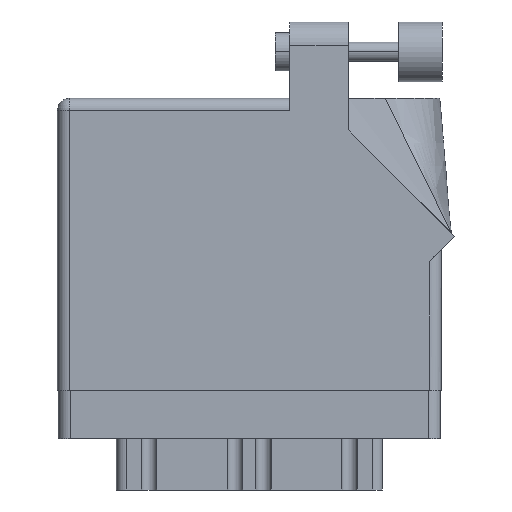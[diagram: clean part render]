
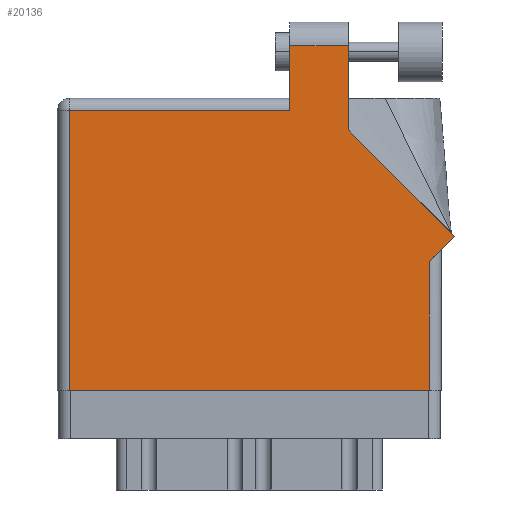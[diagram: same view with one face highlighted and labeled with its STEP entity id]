
A CAD part, front view. The second image highlights one B-rep face of the part: STEP entity #20136.
In plain terms, the highlighted face is planar.
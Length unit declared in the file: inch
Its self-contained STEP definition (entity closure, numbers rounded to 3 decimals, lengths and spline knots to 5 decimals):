
#296 = VERTEX_POINT ( 'NONE', #29452 ) ;
#819 = ORIENTED_EDGE ( 'NONE', *, *, #18401, .T. ) ;
#1143 = PLANE ( 'NONE',  #2238 ) ;
#1325 = VECTOR ( 'NONE', #16028, 39.37008 ) ;
#1350 = DIRECTION ( 'NONE',  ( -1., 0., 0. ) ) ;
#2117 = VECTOR ( 'NONE', #21336, 39.37008 ) ;
#2238 = AXIS2_PLACEMENT_3D ( 'NONE', #15175, #3336, #22206 ) ;
#2289 = CARTESIAN_POINT ( 'NONE',  ( 2.01, 0.737, 0. ) ) ;
#2433 = DIRECTION ( 'NONE',  ( 0., -1., 0. ) ) ;
#3134 = LINE ( 'NONE', #3281, #13833 ) ;
#3281 = CARTESIAN_POINT ( 'NONE',  ( 0., 0., 0. ) ) ;
#3336 = DIRECTION ( 'NONE',  ( 0., 0., -1. ) ) ;
#4710 = CARTESIAN_POINT ( 'NONE',  ( 1.948, 0., 0. ) ) ;
#5114 = ORIENTED_EDGE ( 'NONE', *, *, #14555, .T. ) ;
#5416 = CARTESIAN_POINT ( 'NONE',  ( 1.524, 1.36442, 0. ) ) ;
#7023 = EDGE_CURVE ( 'NONE', #10061, #24584, #21172, .T. ) ;
#7038 = CARTESIAN_POINT ( 'NONE',  ( 1.217, 1.468, 0. ) ) ;
#7581 = ORIENTED_EDGE ( 'NONE', *, *, #28350, .T. ) ;
#8056 = CARTESIAN_POINT ( 'NONE',  ( 1.217, 1.805, 0. ) ) ;
#9410 = LINE ( 'NONE', #28465, #15204 ) ;
#9479 = VERTEX_POINT ( 'NONE', #16394 ) ;
#9563 = DIRECTION ( 'NONE',  ( -1., 0., 0. ) ) ;
#10061 = VERTEX_POINT ( 'NONE', #12580 ) ;
#10605 = DIRECTION ( 'NONE',  ( -0.707, 0.707, 0. ) ) ;
#10945 = EDGE_CURVE ( 'NONE', #30855, #10061, #15712, .T. ) ;
#12081 = LINE ( 'NONE', #16476, #12684 ) ;
#12106 = LINE ( 'NONE', #5416, #21195 ) ;
#12580 = CARTESIAN_POINT ( 'NONE',  ( 1.948, 0.675, 0. ) ) ;
#12672 = FACE_OUTER_BOUND ( 'NONE', #29755, .T. ) ;
#12684 = VECTOR ( 'NONE', #2433, 39.37008 ) ;
#13103 = CARTESIAN_POINT ( 'NONE',  ( 2.08071, 0.80771, 0. ) ) ;
#13833 = VECTOR ( 'NONE', #22327, 39.37008 ) ;
#13899 = ORIENTED_EDGE ( 'NONE', *, *, #26778, .T. ) ;
#14131 = DIRECTION ( 'NONE',  ( 0., -1., 0. ) ) ;
#14555 = EDGE_CURVE ( 'NONE', #25944, #30855, #3134, .T. ) ;
#15175 = CARTESIAN_POINT ( 'NONE',  ( 0., 1.53, 0. ) ) ;
#15204 = VECTOR ( 'NONE', #9563, 39.37008 ) ;
#15604 = LINE ( 'NONE', #13103, #29050 ) ;
#15712 = LINE ( 'NONE', #18375, #1325 ) ;
#16028 = DIRECTION ( 'NONE',  ( 0., 1., 0. ) ) ;
#16394 = CARTESIAN_POINT ( 'NONE',  ( 1.217, 1.805, 0. ) ) ;
#16476 = CARTESIAN_POINT ( 'NONE',  ( 0.062, 0., 0. ) ) ;
#16487 = LINE ( 'NONE', #26012, #23234 ) ;
#17154 = CARTESIAN_POINT ( 'NONE',  ( 1.524, 1.36442, 0. ) ) ;
#17431 = CARTESIAN_POINT ( 'NONE',  ( 1.524, 1.805, 0. ) ) ;
#17796 = EDGE_CURVE ( 'NONE', #24463, #17862, #12106, .T. ) ;
#17862 = VERTEX_POINT ( 'NONE', #17431 ) ;
#17958 = CARTESIAN_POINT ( 'NONE',  ( 2.08071, 0.80771, 0. ) ) ;
#18375 = CARTESIAN_POINT ( 'NONE',  ( 1.948, 0.737, 0. ) ) ;
#18401 = EDGE_CURVE ( 'NONE', #9479, #18559, #16487, .T. ) ;
#18559 = VERTEX_POINT ( 'NONE', #7038 ) ;
#20136 = ADVANCED_FACE ( 'NONE', ( #12672 ), #1143, .F. ) ;
#20399 = LINE ( 'NONE', #8056, #30310 ) ;
#20962 = EDGE_CURVE ( 'NONE', #17862, #9479, #20399, .T. ) ;
#21172 = LINE ( 'NONE', #2289, #2117 ) ;
#21195 = VECTOR ( 'NONE', #21956, 39.37008 ) ;
#21336 = DIRECTION ( 'NONE',  ( 0.707, 0.707, 0. ) ) ;
#21956 = DIRECTION ( 'NONE',  ( 0., 1., 0. ) ) ;
#22110 = CARTESIAN_POINT ( 'NONE',  ( 0.062, 0., 0. ) ) ;
#22206 = DIRECTION ( 'NONE',  ( -1., 0., 0. ) ) ;
#22327 = DIRECTION ( 'NONE',  ( 1., 0., 0. ) ) ;
#23234 = VECTOR ( 'NONE', #14131, 39.37008 ) ;
#23463 = ORIENTED_EDGE ( 'NONE', *, *, #7023, .T. ) ;
#24463 = VERTEX_POINT ( 'NONE', #17154 ) ;
#24584 = VERTEX_POINT ( 'NONE', #17958 ) ;
#24639 = EDGE_CURVE ( 'NONE', #24584, #24463, #15604, .T. ) ;
#25713 = ORIENTED_EDGE ( 'NONE', *, *, #20962, .T. ) ;
#25856 = ORIENTED_EDGE ( 'NONE', *, *, #10945, .T. ) ;
#25882 = ORIENTED_EDGE ( 'NONE', *, *, #17796, .T. ) ;
#25944 = VERTEX_POINT ( 'NONE', #22110 ) ;
#26012 = CARTESIAN_POINT ( 'NONE',  ( 1.217, 1.53, 0. ) ) ;
#26778 = EDGE_CURVE ( 'NONE', #296, #25944, #12081, .T. ) ;
#28350 = EDGE_CURVE ( 'NONE', #18559, #296, #9410, .T. ) ;
#28465 = CARTESIAN_POINT ( 'NONE',  ( 0., 1.468, 0. ) ) ;
#29050 = VECTOR ( 'NONE', #10605, 39.37008 ) ;
#29452 = CARTESIAN_POINT ( 'NONE',  ( 0.062, 1.468, 0. ) ) ;
#29755 = EDGE_LOOP ( 'NONE', ( #25882, #25713, #819, #7581, #13899, #5114, #25856, #23463, #30743 ) ) ;
#30310 = VECTOR ( 'NONE', #1350, 39.37008 ) ;
#30743 = ORIENTED_EDGE ( 'NONE', *, *, #24639, .T. ) ;
#30855 = VERTEX_POINT ( 'NONE', #4710 ) ;
